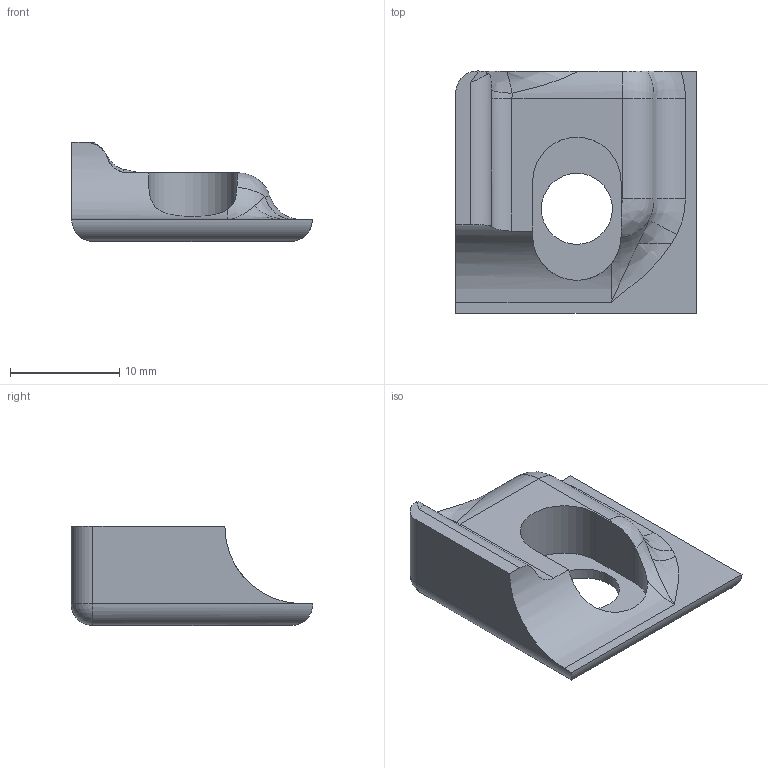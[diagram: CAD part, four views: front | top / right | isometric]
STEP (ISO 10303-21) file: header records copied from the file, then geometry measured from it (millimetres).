
FILE_DESCRIPTION (( 'STEP AP214' ), '1' );
FILE_NAME ('V3_Mag_Release_Cover.STEP', '2013-11-27T07:46:33', ( 'elpi' ), ( '' ), 'SwSTEP 2.0', 'SolidWorks 2013', '' );
FILE_SCHEMA (( 'AUTOMOTIVE_DESIGN' ));
Length unit declared in the file: millimetre
Products named in the file (1): V3_Mag_Release_Cover
Bounding box: 22 x 22.12 x 9.06 mm (x, y, z)
Volume: 1824.6 mm3; surface area: 1422.2 mm2
Topology: 1 solids, 1 shells, 37 faces, 95 edges, 58 vertices
Faces by surface type: cylinder 16, plane 9, bspline 9, torus 2, sphere 1
Entity records: 1597 total; most frequent: CARTESIAN_POINT 758, ORIENTED_EDGE 186, DIRECTION 142, EDGE_CURVE 93, VERTEX_POINT 58, AXIS2_PLACEMENT_3D 53, EDGE_LOOP 39, ADVANCED_FACE 37
